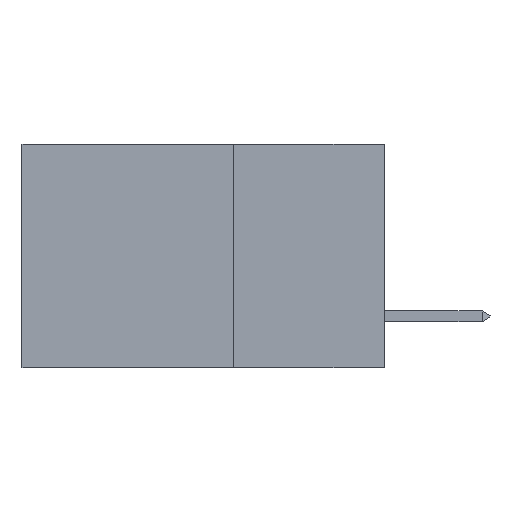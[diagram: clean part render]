
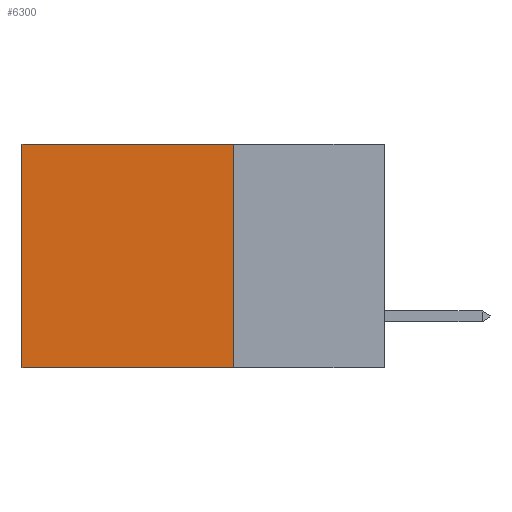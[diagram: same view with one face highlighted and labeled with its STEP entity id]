
A CAD part, left-side view. The second image highlights one B-rep face of the part: STEP entity #6300.
In plain terms, the highlighted planar face has unit normal (-1, 0, 0).
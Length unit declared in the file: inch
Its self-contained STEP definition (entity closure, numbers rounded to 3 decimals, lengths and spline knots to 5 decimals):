
#522 = EDGE_CURVE ( 'NONE', #10920, #10272, #10382, .T. ) ;
#603 = CARTESIAN_POINT ( 'NONE',  ( 0.2875, 0.6, 0. ) ) ;
#1359 = EDGE_CURVE ( 'NONE', #22039, #10920, #3495, .T. ) ;
#3495 = LINE ( 'NONE', #10411, #14330 ) ;
#5290 = CARTESIAN_POINT ( 'NONE',  ( 0.2875, 0.6, -0.37 ) ) ;
#6300 = ADVANCED_FACE ( 'NONE', ( #20422 ), #14923, .F. ) ;
#6883 = CARTESIAN_POINT ( 'NONE',  ( 0.2875, 0.6, 0. ) ) ;
#7704 = EDGE_CURVE ( 'NONE', #22039, #18441, #15591, .T. ) ;
#7858 = ORIENTED_EDGE ( 'NONE', *, *, #7704, .T. ) ;
#8686 = CARTESIAN_POINT ( 'NONE',  ( 0.2875, 0.25, -0.37 ) ) ;
#9570 = EDGE_LOOP ( 'NONE', ( #10457, #19526, #13437, #7858 ) ) ;
#10272 = VERTEX_POINT ( 'NONE', #5290 ) ;
#10382 = LINE ( 'NONE', #8686, #16265 ) ;
#10411 = CARTESIAN_POINT ( 'NONE',  ( 0.2875, 0.25, 0. ) ) ;
#10457 = ORIENTED_EDGE ( 'NONE', *, *, #12857, .T. ) ;
#10760 = DIRECTION ( 'NONE',  ( 0., 1., 0. ) ) ;
#10920 = VERTEX_POINT ( 'NONE', #18189 ) ;
#11763 = CARTESIAN_POINT ( 'NONE',  ( 0.2875, 0.25, 0. ) ) ;
#11990 = CARTESIAN_POINT ( 'NONE',  ( 0.2875, 0.25, 0. ) ) ;
#12857 = EDGE_CURVE ( 'NONE', #18441, #10272, #15228, .T. ) ;
#13118 = DIRECTION ( 'NONE',  ( 0., 0., -1. ) ) ;
#13437 = ORIENTED_EDGE ( 'NONE', *, *, #1359, .F. ) ;
#13642 = DIRECTION ( 'NONE',  ( 0., 0., -1. ) ) ;
#13769 = AXIS2_PLACEMENT_3D ( 'NONE', #11763, #21778, #13118 ) ;
#14222 = DIRECTION ( 'NONE',  ( 0., 0., -1. ) ) ;
#14330 = VECTOR ( 'NONE', #14222, 39.37008 ) ;
#14923 = PLANE ( 'NONE',  #13769 ) ;
#15228 = LINE ( 'NONE', #6883, #21351 ) ;
#15546 = DIRECTION ( 'NONE',  ( 0., 1., 0. ) ) ;
#15579 = CARTESIAN_POINT ( 'NONE',  ( 0.2875, 0.25, 0. ) ) ;
#15591 = LINE ( 'NONE', #11990, #18737 ) ;
#16265 = VECTOR ( 'NONE', #15546, 39.37008 ) ;
#18189 = CARTESIAN_POINT ( 'NONE',  ( 0.2875, 0.25, -0.37 ) ) ;
#18441 = VERTEX_POINT ( 'NONE', #603 ) ;
#18737 = VECTOR ( 'NONE', #10760, 39.37008 ) ;
#19526 = ORIENTED_EDGE ( 'NONE', *, *, #522, .F. ) ;
#20422 = FACE_OUTER_BOUND ( 'NONE', #9570, .T. ) ;
#21351 = VECTOR ( 'NONE', #13642, 39.37008 ) ;
#21778 = DIRECTION ( 'NONE',  ( 1., 0., 0. ) ) ;
#22039 = VERTEX_POINT ( 'NONE', #15579 ) ;
